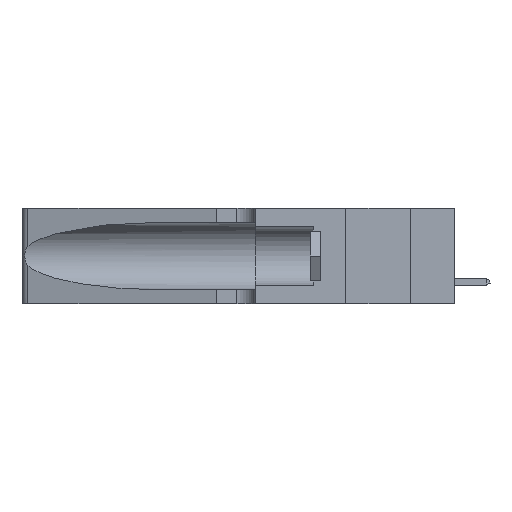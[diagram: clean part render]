
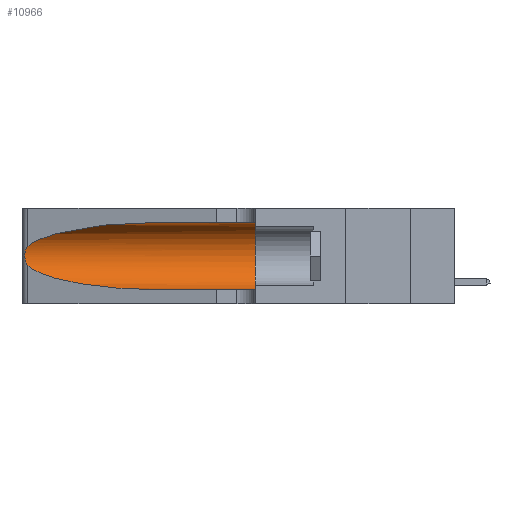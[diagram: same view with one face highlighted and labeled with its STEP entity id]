
A CAD part, left-side view. The second image highlights one B-rep face of the part: STEP entity #10966.
In plain terms, the highlighted cylindrical face has radius 3.308 mm (diameter 6.617 mm), a partial arc.
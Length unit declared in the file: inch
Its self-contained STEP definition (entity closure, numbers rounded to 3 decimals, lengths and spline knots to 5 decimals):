
#204 = ORIENTED_EDGE ( 'NONE', *, *, #8597, .F. ) ;
#279 = CARTESIAN_POINT ( 'NONE',  ( 0.1305, 0.35, 0.31525 ) ) ;
#410 = DIRECTION ( 'NONE',  ( 0., 1., 0. ) ) ;
#496 = CARTESIAN_POINT ( 'NONE',  ( 0.25555, 1.22993, 0.14849 ) ) ;
#760 = CARTESIAN_POINT ( 'NONE',  ( 0.25487, 1.22718, 0.14631 ) ) ;
#1856 = CARTESIAN_POINT ( 'NONE',  ( 0.1305, 0.72297, 0.05475 ) ) ;
#2365 = CARTESIAN_POINT ( 'NONE',  ( 0.26075, 1.23896, 0.19203 ) ) ;
#2493 = CARTESIAN_POINT ( 'NONE',  ( 0.18966, 0.96281, 0.05475 ) ) ;
#2772 = CYLINDRICAL_SURFACE ( 'NONE', #9607, 0.13025 ) ;
#3981 = LINE ( 'NONE', #24992, #25190 ) ;
#4067 = EDGE_CURVE ( 'NONE', #25196, #15211, #3981, .T. ) ;
#4885 = CARTESIAN_POINT ( 'NONE',  ( 0.26017, 1.23833, 0.17102 ) ) ;
#5093 = ORIENTED_EDGE ( 'NONE', *, *, #4067, .T. ) ;
#6549 = CARTESIAN_POINT ( 'NONE',  ( 0.26018, 1.23835, 0.19895 ) ) ;
#6598 = VECTOR ( 'NONE', #23208, 39.37008 ) ;
#6978 =( BOUNDED_CURVE ( )  B_SPLINE_CURVE ( 3, ( #12170, #7748, #26025, #19199 ),
 .UNSPECIFIED., .F., .T. ) 
 B_SPLINE_CURVE_WITH_KNOTS ( ( 4, 4 ),
 ( 1.5708, 2.84003 ),
 .UNSPECIFIED. ) 
 CURVE ( )  GEOMETRIC_REPRESENTATION_ITEM ( )  RATIONAL_B_SPLINE_CURVE ( ( 1., 0.87, 0.87, 1. ) ) 
 REPRESENTATION_ITEM ( '' )  );
#7303 = CARTESIAN_POINT ( 'NONE',  ( 0.25639, 1.23186, 0.15144 ) ) ;
#7748 = CARTESIAN_POINT ( 'NONE',  ( 0.18966, 0.96281, 0.31525 ) ) ;
#7799 = AXIS2_PLACEMENT_3D ( 'NONE', #14225, #410, #19189 ) ;
#8597 = EDGE_CURVE ( 'NONE', #24530, #26026, #20108, .T. ) ;
#8691 = ORIENTED_EDGE ( 'NONE', *, *, #25773, .T. ) ;
#8911 = CARTESIAN_POINT ( 'NONE',  ( 0.25487, 1.22718, 0.22369 ) ) ;
#9236 =( BOUNDED_CURVE ( )  B_SPLINE_CURVE ( 3, ( #28508, #16498, #2493, #28212 ),
 .UNSPECIFIED., .F., .F. ) 
 B_SPLINE_CURVE_WITH_KNOTS ( ( 4, 4 ),
 ( 3.44316, 4.71239 ),
 .UNSPECIFIED. ) 
 CURVE ( )  GEOMETRIC_REPRESENTATION_ITEM ( )  RATIONAL_B_SPLINE_CURVE ( ( 1., 0.87, 0.87, 1. ) ) 
 REPRESENTATION_ITEM ( '' )  );
#9607 = AXIS2_PLACEMENT_3D ( 'NONE', #15934, #29986, #22728 ) ;
#9755 = CARTESIAN_POINT ( 'NONE',  ( 0.25856, 1.23593, 0.16098 ) ) ;
#10966 = ADVANCED_FACE ( 'NONE', ( #13034 ), #2772, .F. ) ;
#11258 = ORIENTED_EDGE ( 'NONE', *, *, #15056, .T. ) ;
#12141 = CARTESIAN_POINT ( 'NONE',  ( 0.25789, 1.23486, 0.15765 ) ) ;
#12170 = CARTESIAN_POINT ( 'NONE',  ( 0.1305, 0.72297, 0.31525 ) ) ;
#12408 = CARTESIAN_POINT ( 'NONE',  ( 0.25787, 1.23484, 0.2124 ) ) ;
#13034 = FACE_OUTER_BOUND ( 'NONE', #26400, .T. ) ;
#13967 = ORIENTED_EDGE ( 'NONE', *, *, #14644, .T. ) ;
#14225 = CARTESIAN_POINT ( 'NONE',  ( 0.1305, 0.35, 0.185 ) ) ;
#14644 = EDGE_CURVE ( 'NONE', #27517, #25196, #9236, .T. ) ;
#15056 = EDGE_CURVE ( 'NONE', #24530, #21455, #6978, .T. ) ;
#15211 = VERTEX_POINT ( 'NONE', #17547 ) ;
#15801 = ORIENTED_EDGE ( 'NONE', *, *, #20745, .F. ) ;
#15934 = CARTESIAN_POINT ( 'NONE',  ( 0.1305, 1.61858, 0.185 ) ) ;
#16498 = CARTESIAN_POINT ( 'NONE',  ( 0.2373, 1.15595, 0.08982 ) ) ;
#17547 = CARTESIAN_POINT ( 'NONE',  ( 0.1305, 0.35, 0.05475 ) ) ;
#18524 = CARTESIAN_POINT ( 'NONE',  ( 0.1305, 1.61858, 0.31525 ) ) ;
#19022 = CARTESIAN_POINT ( 'NONE',  ( 0.25639, 1.23184, 0.21858 ) ) ;
#19189 = DIRECTION ( 'NONE',  ( 0., 0., 1. ) ) ;
#19199 = CARTESIAN_POINT ( 'NONE',  ( 0.25487, 1.22718, 0.22369 ) ) ;
#20108 = LINE ( 'NONE', #18524, #6598 ) ;
#20389 = DIRECTION ( 'NONE',  ( 0., -1., 0. ) ) ;
#20545 = CARTESIAN_POINT ( 'NONE',  ( 0.25854, 1.2359, 0.20912 ) ) ;
#20745 = EDGE_CURVE ( 'NONE', #26026, #15211, #27337, .T. ) ;
#21455 = VERTEX_POINT ( 'NONE', #8911 ) ;
#21911 = CARTESIAN_POINT ( 'NONE',  ( 0.25487, 1.22718, 0.22369 ) ) ;
#22728 = DIRECTION ( 'NONE',  ( 0., 0., -1. ) ) ;
#23208 = DIRECTION ( 'NONE',  ( 0., -1., 0. ) ) ;
#24259 = CARTESIAN_POINT ( 'NONE',  ( 0.25555, 1.22994, 0.2215 ) ) ;
#24530 = VERTEX_POINT ( 'NONE', #29496 ) ;
#24605 = B_SPLINE_CURVE_WITH_KNOTS ( 'NONE', 3,
 ( #21911, #24259, #19022, #12408, #20545, #6549, #2365, #28046, #4885, #9755, #12141, #7303, #496, #25892 ),
 .UNSPECIFIED., .F., .F.,
 ( 4, 2, 2, 2, 2, 2, 4 ),
 ( 0., 0.00027, 0.00053, 0.00107, 0.0016, 0.00187, 0.00214 ),
 .UNSPECIFIED. ) ;
#24992 = CARTESIAN_POINT ( 'NONE',  ( 0.1305, 1.61858, 0.05475 ) ) ;
#25190 = VECTOR ( 'NONE', #20389, 39.37008 ) ;
#25196 = VERTEX_POINT ( 'NONE', #1856 ) ;
#25773 = EDGE_CURVE ( 'NONE', #21455, #27517, #24605, .T. ) ;
#25892 = CARTESIAN_POINT ( 'NONE',  ( 0.25487, 1.22718, 0.14631 ) ) ;
#26025 = CARTESIAN_POINT ( 'NONE',  ( 0.2373, 1.15595, 0.28018 ) ) ;
#26026 = VERTEX_POINT ( 'NONE', #279 ) ;
#26400 = EDGE_LOOP ( 'NONE', ( #11258, #8691, #13967, #5093, #15801, #204 ) ) ;
#27337 = CIRCLE ( 'NONE', #7799, 0.13025 ) ;
#27517 = VERTEX_POINT ( 'NONE', #760 ) ;
#28046 = CARTESIAN_POINT ( 'NONE',  ( 0.26075, 1.23896, 0.178 ) ) ;
#28212 = CARTESIAN_POINT ( 'NONE',  ( 0.1305, 0.72297, 0.05475 ) ) ;
#28508 = CARTESIAN_POINT ( 'NONE',  ( 0.25487, 1.22718, 0.14631 ) ) ;
#29496 = CARTESIAN_POINT ( 'NONE',  ( 0.1305, 0.72297, 0.31525 ) ) ;
#29986 = DIRECTION ( 'NONE',  ( 0., -1., 0. ) ) ;
